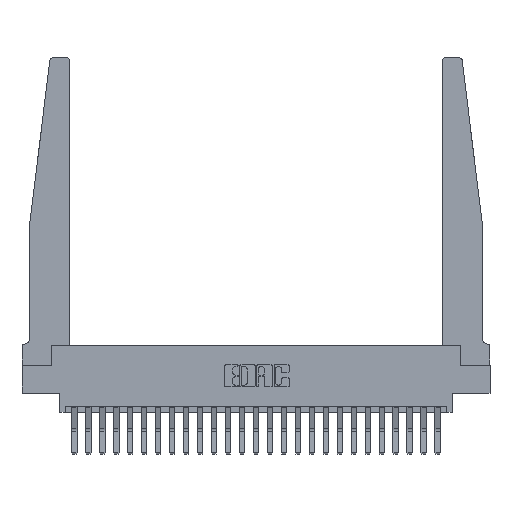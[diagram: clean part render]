
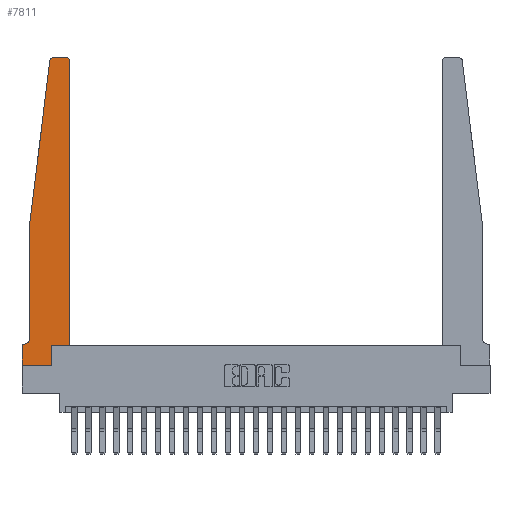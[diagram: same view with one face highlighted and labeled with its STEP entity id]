
A CAD part, top view. The second image highlights one B-rep face of the part: STEP entity #7811.
In plain terms, the highlighted planar face has unit normal (0, 0, 1).
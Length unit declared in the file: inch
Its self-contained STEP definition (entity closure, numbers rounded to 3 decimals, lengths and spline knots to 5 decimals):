
#274 = ORIENTED_EDGE ( 'NONE', *, *, #20889, .T. ) ;
#360 = VECTOR ( 'NONE', #5328, 39.37008 ) ;
#591 = VERTEX_POINT ( 'NONE', #10004 ) ;
#721 = EDGE_CURVE ( 'NONE', #10631, #591, #1701, .T. ) ;
#1182 = VECTOR ( 'NONE', #5066, 39.37008 ) ;
#1329 = VECTOR ( 'NONE', #4528, 39.37008 ) ;
#1701 = CIRCLE ( 'NONE', #20313, 0.03 ) ;
#1709 = VERTEX_POINT ( 'NONE', #8213 ) ;
#1826 = EDGE_CURVE ( 'NONE', #21321, #14424, #18989, .T. ) ;
#1890 = VECTOR ( 'NONE', #24567, 39.37008 ) ;
#1936 = ORIENTED_EDGE ( 'NONE', *, *, #12769, .T. ) ;
#2368 = CARTESIAN_POINT ( 'NONE',  ( 0.425, 2.72, 0.37 ) ) ;
#2420 = EDGE_LOOP ( 'NONE', ( #24153, #23702, #3469, #14979, #5202, #1936, #14094, #4064, #23075, #274, #4653, #10497 ) ) ;
#2493 = CARTESIAN_POINT ( 'NONE',  ( 0.27653, 2.75, 0.37 ) ) ;
#2578 = AXIS2_PLACEMENT_3D ( 'NONE', #21795, #10401, #23663 ) ;
#3469 = ORIENTED_EDGE ( 'NONE', *, *, #3912, .T. ) ;
#3729 = AXIS2_PLACEMENT_3D ( 'NONE', #19386, #4193, #17580 ) ;
#3740 = VECTOR ( 'NONE', #14217, 39.37008 ) ;
#3910 = AXIS2_PLACEMENT_3D ( 'NONE', #20299, #8889, #22166 ) ;
#3912 = EDGE_CURVE ( 'NONE', #591, #21321, #11418, .T. ) ;
#4064 = ORIENTED_EDGE ( 'NONE', *, *, #16405, .T. ) ;
#4135 = VERTEX_POINT ( 'NONE', #6263 ) ;
#4148 = VERTEX_POINT ( 'NONE', #12009 ) ;
#4187 = CARTESIAN_POINT ( 'NONE',  ( 0.425, 0.18, 0.37 ) ) ;
#4193 = DIRECTION ( 'NONE',  ( 0., 0., 1. ) ) ;
#4214 = FACE_OUTER_BOUND ( 'NONE', #2420, .T. ) ;
#4528 = DIRECTION ( 'NONE',  ( -1., 0., 0. ) ) ;
#4620 = VERTEX_POINT ( 'NONE', #24557 ) ;
#4653 = ORIENTED_EDGE ( 'NONE', *, *, #24626, .T. ) ;
#4729 = DIRECTION ( 'NONE',  ( 0., 0., 1. ) ) ;
#4741 = LINE ( 'NONE', #8452, #14913 ) ;
#5066 = DIRECTION ( 'NONE',  ( 0., 1., 0. ) ) ;
#5202 = ORIENTED_EDGE ( 'NONE', *, *, #16106, .T. ) ;
#5328 = DIRECTION ( 'NONE',  ( 0., 1., 0. ) ) ;
#6030 = VERTEX_POINT ( 'NONE', #23954 ) ;
#6263 = CARTESIAN_POINT ( 'NONE',  ( 0.2605, 0.18, 0.37 ) ) ;
#6463 = CARTESIAN_POINT ( 'NONE',  ( 0.065, 0.1875, 0.37 ) ) ;
#6843 = EDGE_CURVE ( 'NONE', #1709, #4135, #21855, .T. ) ;
#6961 = VECTOR ( 'NONE', #24500, 39.37008 ) ;
#7811 = ADVANCED_FACE ( 'NONE', ( #4214 ), #13740, .T. ) ;
#8064 = CARTESIAN_POINT ( 'NONE',  ( 0.015, 0.1875, 0.37 ) ) ;
#8213 = CARTESIAN_POINT ( 'NONE',  ( 0.2605, 0., 0.37 ) ) ;
#8452 = CARTESIAN_POINT ( 'NONE',  ( 0.25, 2.75, 0.37 ) ) ;
#8889 = DIRECTION ( 'NONE',  ( 0., 0., 1. ) ) ;
#9165 = CARTESIAN_POINT ( 'NONE',  ( 0.2605, 0.18, 0.37 ) ) ;
#9270 = CARTESIAN_POINT ( 'NONE',  ( 0.065, 1.25, 0.37 ) ) ;
#9347 = CARTESIAN_POINT ( 'NONE',  ( 0.065, 1.25, 0.37 ) ) ;
#9721 = EDGE_CURVE ( 'NONE', #16613, #4620, #14299, .T. ) ;
#10004 = CARTESIAN_POINT ( 'NONE',  ( 0.24675, 2.72367, 0.37 ) ) ;
#10401 = DIRECTION ( 'NONE',  ( 0., 0., -1. ) ) ;
#10497 = ORIENTED_EDGE ( 'NONE', *, *, #9721, .T. ) ;
#10631 = VERTEX_POINT ( 'NONE', #2493 ) ;
#11139 = DIRECTION ( 'NONE',  ( 1., 0., 0. ) ) ;
#11381 = VECTOR ( 'NONE', #11139, 39.37008 ) ;
#11418 = LINE ( 'NONE', #9347, #6961 ) ;
#11584 = VERTEX_POINT ( 'NONE', #16655 ) ;
#11989 = LINE ( 'NONE', #20735, #11381 ) ;
#12009 = CARTESIAN_POINT ( 'NONE',  ( 0.425, 0.18, 0.37 ) ) ;
#12078 = LINE ( 'NONE', #13278, #1890 ) ;
#12227 = VECTOR ( 'NONE', #19463, 39.37008 ) ;
#12769 = EDGE_CURVE ( 'NONE', #14775, #6030, #16606, .T. ) ;
#13278 = CARTESIAN_POINT ( 'NONE',  ( 0., 0., 0.37 ) ) ;
#13718 = EDGE_CURVE ( 'NONE', #6030, #11584, #12078, .T. ) ;
#13740 = PLANE ( 'NONE',  #3729 ) ;
#14094 = ORIENTED_EDGE ( 'NONE', *, *, #13718, .T. ) ;
#14100 = CIRCLE ( 'NONE', #2578, 0.05 ) ;
#14217 = DIRECTION ( 'NONE',  ( 0., -1., 0. ) ) ;
#14299 = CIRCLE ( 'NONE', #3910, 0.03 ) ;
#14424 = VERTEX_POINT ( 'NONE', #19137 ) ;
#14775 = VERTEX_POINT ( 'NONE', #8064 ) ;
#14913 = VECTOR ( 'NONE', #21753, 39.37008 ) ;
#14979 = ORIENTED_EDGE ( 'NONE', *, *, #1826, .T. ) ;
#16106 = EDGE_CURVE ( 'NONE', #14424, #14775, #14100, .T. ) ;
#16162 = CARTESIAN_POINT ( 'NONE',  ( 0.27653, 2.72, 0.37 ) ) ;
#16405 = EDGE_CURVE ( 'NONE', #11584, #1709, #11989, .T. ) ;
#16606 = LINE ( 'NONE', #6463, #1329 ) ;
#16613 = VERTEX_POINT ( 'NONE', #2368 ) ;
#16655 = CARTESIAN_POINT ( 'NONE',  ( 0., 0., 0.37 ) ) ;
#17580 = DIRECTION ( 'NONE',  ( 1., 0., 0. ) ) ;
#17912 = LINE ( 'NONE', #4187, #12227 ) ;
#18100 = DIRECTION ( 'NONE',  ( 1., 0., 0. ) ) ;
#18989 = LINE ( 'NONE', #19881, #3740 ) ;
#19137 = CARTESIAN_POINT ( 'NONE',  ( 0.065, 0.2375, 0.37 ) ) ;
#19386 = CARTESIAN_POINT ( 'NONE',  ( 0., 0.1875, 0.37 ) ) ;
#19463 = DIRECTION ( 'NONE',  ( 1., 0., 0. ) ) ;
#19881 = CARTESIAN_POINT ( 'NONE',  ( 0.065, 1.25, 0.37 ) ) ;
#20299 = CARTESIAN_POINT ( 'NONE',  ( 0.395, 2.72, 0.37 ) ) ;
#20313 = AXIS2_PLACEMENT_3D ( 'NONE', #16162, #4729, #18100 ) ;
#20735 = CARTESIAN_POINT ( 'NONE',  ( 0., 0., 0.37 ) ) ;
#20889 = EDGE_CURVE ( 'NONE', #4135, #4148, #17912, .T. ) ;
#21025 = EDGE_CURVE ( 'NONE', #4620, #10631, #4741, .T. ) ;
#21321 = VERTEX_POINT ( 'NONE', #9270 ) ;
#21495 = LINE ( 'NONE', #22104, #1182 ) ;
#21753 = DIRECTION ( 'NONE',  ( -1., 0., 0. ) ) ;
#21795 = CARTESIAN_POINT ( 'NONE',  ( 0.015, 0.2375, 0.37 ) ) ;
#21855 = LINE ( 'NONE', #9165, #360 ) ;
#22104 = CARTESIAN_POINT ( 'NONE',  ( 0.425, 0.18, 0.37 ) ) ;
#22166 = DIRECTION ( 'NONE',  ( 1., 0., 0. ) ) ;
#23075 = ORIENTED_EDGE ( 'NONE', *, *, #6843, .T. ) ;
#23663 = DIRECTION ( 'NONE',  ( -1., 0., 0. ) ) ;
#23702 = ORIENTED_EDGE ( 'NONE', *, *, #721, .T. ) ;
#23954 = CARTESIAN_POINT ( 'NONE',  ( 0., 0.1875, 0.37 ) ) ;
#24153 = ORIENTED_EDGE ( 'NONE', *, *, #21025, .T. ) ;
#24500 = DIRECTION ( 'NONE',  ( -0.122, -0.992, 0. ) ) ;
#24557 = CARTESIAN_POINT ( 'NONE',  ( 0.395, 2.75, 0.37 ) ) ;
#24567 = DIRECTION ( 'NONE',  ( 0., -1., 0. ) ) ;
#24626 = EDGE_CURVE ( 'NONE', #4148, #16613, #21495, .T. ) ;
